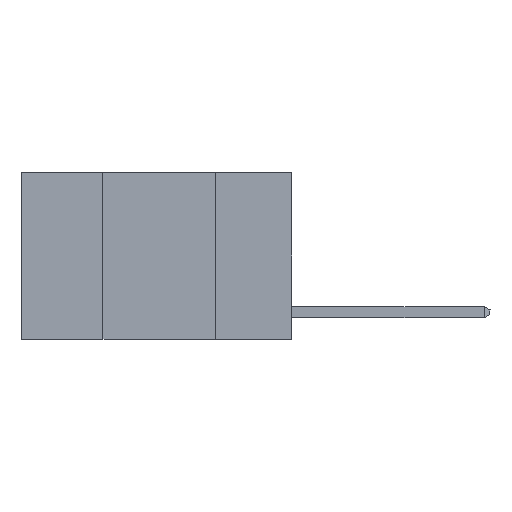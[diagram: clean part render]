
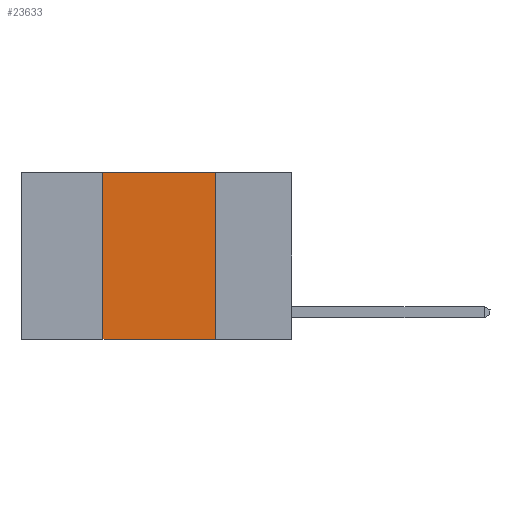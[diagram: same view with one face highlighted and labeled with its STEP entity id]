
A CAD part, left-side view. The second image highlights one B-rep face of the part: STEP entity #23633.
In plain terms, the highlighted planar face has unit normal (-1, 0, 0).
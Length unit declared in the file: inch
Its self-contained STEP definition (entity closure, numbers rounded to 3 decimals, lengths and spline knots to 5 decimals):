
#252 = EDGE_CURVE ( 'NONE', #19491, #23239, #7638, .T. ) ;
#815 = EDGE_CURVE ( 'NONE', #8560, #23239, #4048, .T. ) ;
#2568 = ORIENTED_EDGE ( 'NONE', *, *, #5254, .F. ) ;
#2875 = ORIENTED_EDGE ( 'NONE', *, *, #26057, .F. ) ;
#3914 = VECTOR ( 'NONE', #15253, 39.37008 ) ;
#4048 = LINE ( 'NONE', #22819, #15893 ) ;
#5254 = EDGE_CURVE ( 'NONE', #24034, #8560, #24097, .T. ) ;
#7188 = CARTESIAN_POINT ( 'NONE',  ( 0., 0.6, 0. ) ) ;
#7638 = LINE ( 'NONE', #10188, #24539 ) ;
#8560 = VERTEX_POINT ( 'NONE', #19972 ) ;
#9247 = ORIENTED_EDGE ( 'NONE', *, *, #252, .T. ) ;
#9793 = AXIS2_PLACEMENT_3D ( 'NONE', #7188, #11751, #27100 ) ;
#9896 = LINE ( 'NONE', #10823, #3914 ) ;
#10188 = CARTESIAN_POINT ( 'NONE',  ( 0., 0.6, -0.37 ) ) ;
#10823 = CARTESIAN_POINT ( 'NONE',  ( 0., 0.42, 0. ) ) ;
#11751 = DIRECTION ( 'NONE',  ( 1., 0., 0. ) ) ;
#12172 = EDGE_LOOP ( 'NONE', ( #16410, #2568, #2875, #9247 ) ) ;
#12378 = VECTOR ( 'NONE', #28189, 39.37008 ) ;
#12427 = CARTESIAN_POINT ( 'NONE',  ( 0., 0.17, -0.37 ) ) ;
#15079 = CARTESIAN_POINT ( 'NONE',  ( 0., 0.6, 0. ) ) ;
#15253 = DIRECTION ( 'NONE',  ( 0., 0., 1. ) ) ;
#15893 = VECTOR ( 'NONE', #22642, 39.37008 ) ;
#16410 = ORIENTED_EDGE ( 'NONE', *, *, #815, .F. ) ;
#19491 = VERTEX_POINT ( 'NONE', #22218 ) ;
#19972 = CARTESIAN_POINT ( 'NONE',  ( 0., 0.17, 0. ) ) ;
#22218 = CARTESIAN_POINT ( 'NONE',  ( 0., 0.42, -0.37 ) ) ;
#22642 = DIRECTION ( 'NONE',  ( 0., 0., -1. ) ) ;
#22819 = CARTESIAN_POINT ( 'NONE',  ( 0., 0.17, 0. ) ) ;
#23239 = VERTEX_POINT ( 'NONE', #12427 ) ;
#23633 = ADVANCED_FACE ( 'NONE', ( #27510 ), #24917, .F. ) ;
#24034 = VERTEX_POINT ( 'NONE', #26043 ) ;
#24097 = LINE ( 'NONE', #15079, #12378 ) ;
#24539 = VECTOR ( 'NONE', #24820, 39.37008 ) ;
#24820 = DIRECTION ( 'NONE',  ( 0., -1., 0. ) ) ;
#24917 = PLANE ( 'NONE',  #9793 ) ;
#26043 = CARTESIAN_POINT ( 'NONE',  ( 0., 0.42, 0. ) ) ;
#26057 = EDGE_CURVE ( 'NONE', #19491, #24034, #9896, .T. ) ;
#27100 = DIRECTION ( 'NONE',  ( 0., 0., -1. ) ) ;
#27510 = FACE_OUTER_BOUND ( 'NONE', #12172, .T. ) ;
#28189 = DIRECTION ( 'NONE',  ( 0., -1., 0. ) ) ;
